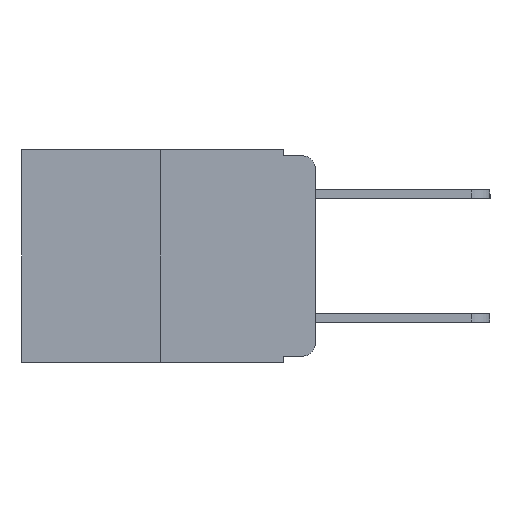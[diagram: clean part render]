
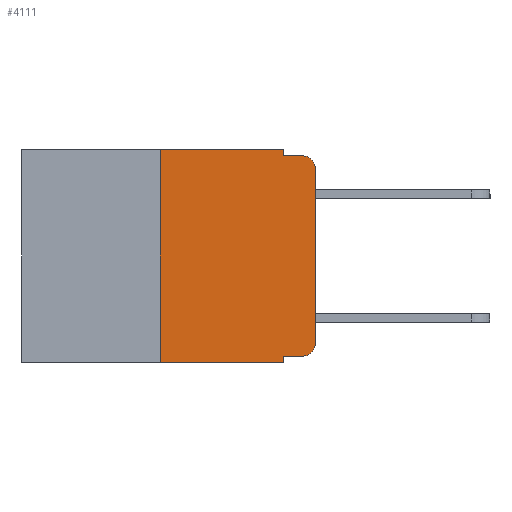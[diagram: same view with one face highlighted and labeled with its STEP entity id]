
A CAD part, left-side view. The second image highlights one B-rep face of the part: STEP entity #4111.
In plain terms, the highlighted planar face has unit normal (-1, 0, 0).
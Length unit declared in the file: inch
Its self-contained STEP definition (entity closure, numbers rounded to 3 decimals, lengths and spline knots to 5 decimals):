
#1461 = ORIENTED_EDGE ( 'NONE', *, *, #3324, .T. ) ;
#2060 = CARTESIAN_POINT ( 'NONE',  ( 0., 0.473, 0. ) ) ;
#2129 = VERTEX_POINT ( 'NONE', #2638 ) ;
#2429 = EDGE_CURVE ( 'NONE', #4318, #19544, #10494, .T. ) ;
#2447 = CARTESIAN_POINT ( 'NONE',  ( 0., 0.25, 0. ) ) ;
#2461 = ORIENTED_EDGE ( 'NONE', *, *, #3360, .F. ) ;
#2638 = CARTESIAN_POINT ( 'NONE',  ( 0., 0.02, -0.01 ) ) ;
#2941 = EDGE_CURVE ( 'NONE', #18041, #9579, #5008, .T. ) ;
#3286 = EDGE_CURVE ( 'NONE', #7197, #5409, #10718, .T. ) ;
#3324 = EDGE_CURVE ( 'NONE', #5409, #2129, #13878, .T. ) ;
#3356 = EDGE_CURVE ( 'NONE', #8829, #2129, #12909, .T. ) ;
#3360 = EDGE_CURVE ( 'NONE', #19544, #8829, #9157, .T. ) ;
#3364 = EDGE_CURVE ( 'NONE', #18041, #4318, #12422, .T. ) ;
#3393 = EDGE_CURVE ( 'NONE', #12695, #9579, #19845, .T. ) ;
#3397 = EDGE_CURVE ( 'NONE', #12695, #16929, #7543, .T. ) ;
#3403 = EDGE_CURVE ( 'NONE', #16929, #7197, #15535, .T. ) ;
#3817 = VECTOR ( 'NONE', #18798, 39.37008 ) ;
#4111 = ADVANCED_FACE ( 'NONE', ( #17070 ), #15646, .F. ) ;
#4318 = VERTEX_POINT ( 'NONE', #20542 ) ;
#4374 = EDGE_LOOP ( 'NONE', ( #9248, #1461, #4467, #2461, #11965, #5166, #5880, #7591, #19672, #5040 ) ) ;
#4393 = CARTESIAN_POINT ( 'NONE',  ( 0., 0.051, -0.01 ) ) ;
#4467 = ORIENTED_EDGE ( 'NONE', *, *, #3356, .F. ) ;
#4569 = CARTESIAN_POINT ( 'NONE',  ( 0., 0.051, 0. ) ) ;
#5008 = LINE ( 'NONE', #8054, #17343 ) ;
#5040 = ORIENTED_EDGE ( 'NONE', *, *, #3403, .T. ) ;
#5166 = ORIENTED_EDGE ( 'NONE', *, *, #3364, .F. ) ;
#5409 = VERTEX_POINT ( 'NONE', #11199 ) ;
#5774 = DIRECTION ( 'NONE',  ( 0., -1., 0. ) ) ;
#5880 = ORIENTED_EDGE ( 'NONE', *, *, #2941, .T. ) ;
#5908 = DIRECTION ( 'NONE',  ( 1., 0., 0. ) ) ;
#5954 = DIRECTION ( 'NONE',  ( 0., 0., 1. ) ) ;
#6114 = DIRECTION ( 'NONE',  ( -1., 0., 0. ) ) ;
#7197 = VERTEX_POINT ( 'NONE', #17632 ) ;
#7543 = LINE ( 'NONE', #8169, #19384 ) ;
#7591 = ORIENTED_EDGE ( 'NONE', *, *, #3393, .F. ) ;
#8025 = DIRECTION ( 'NONE',  ( 0., 0., 1. ) ) ;
#8054 = CARTESIAN_POINT ( 'NONE',  ( 0., 0.473, -0.343 ) ) ;
#8056 = VECTOR ( 'NONE', #8025, 39.37008 ) ;
#8169 = CARTESIAN_POINT ( 'NONE',  ( 0., 0.051, -0.333 ) ) ;
#8247 = DIRECTION ( 'NONE',  ( -1., 0., 0. ) ) ;
#8829 = VERTEX_POINT ( 'NONE', #20942 ) ;
#9157 = LINE ( 'NONE', #12878, #3817 ) ;
#9248 = ORIENTED_EDGE ( 'NONE', *, *, #3286, .T. ) ;
#9579 = VERTEX_POINT ( 'NONE', #18326 ) ;
#9850 = AXIS2_PLACEMENT_3D ( 'NONE', #17580, #8247, #19045 ) ;
#9942 = DIRECTION ( 'NONE',  ( 0., -1., 0. ) ) ;
#10494 = LINE ( 'NONE', #10959, #14647 ) ;
#10718 = LINE ( 'NONE', #15676, #18728 ) ;
#10959 = CARTESIAN_POINT ( 'NONE',  ( 0., 0.473, 0. ) ) ;
#11199 = CARTESIAN_POINT ( 'NONE',  ( 0., 0., -0.03 ) ) ;
#11469 = DIRECTION ( 'NONE',  ( 0., 0., -1. ) ) ;
#11965 = ORIENTED_EDGE ( 'NONE', *, *, #2429, .F. ) ;
#12422 = LINE ( 'NONE', #2447, #8056 ) ;
#12592 = CARTESIAN_POINT ( 'NONE',  ( 0., 0.051, 0. ) ) ;
#12695 = VERTEX_POINT ( 'NONE', #20252 ) ;
#12878 = CARTESIAN_POINT ( 'NONE',  ( 0., 0.051, 0. ) ) ;
#12884 = AXIS2_PLACEMENT_3D ( 'NONE', #2060, #5908, #17093 ) ;
#12909 = LINE ( 'NONE', #4393, #20702 ) ;
#13878 = CIRCLE ( 'NONE', #16419, 0.02 ) ;
#14647 = VECTOR ( 'NONE', #5774, 39.37008 ) ;
#15535 = CIRCLE ( 'NONE', #9850, 0.02 ) ;
#15646 = PLANE ( 'NONE',  #12884 ) ;
#15676 = CARTESIAN_POINT ( 'NONE',  ( 0., 0., 0. ) ) ;
#15806 = CARTESIAN_POINT ( 'NONE',  ( 0., 0.02, -0.03 ) ) ;
#15926 = DIRECTION ( 'NONE',  ( 0., -1., 0. ) ) ;
#15949 = DIRECTION ( 'NONE',  ( 0., -1., 0. ) ) ;
#15990 = VECTOR ( 'NONE', #11469, 39.37008 ) ;
#16102 = CARTESIAN_POINT ( 'NONE',  ( 0., 0.25, -0.343 ) ) ;
#16419 = AXIS2_PLACEMENT_3D ( 'NONE', #15806, #6114, #17256 ) ;
#16929 = VERTEX_POINT ( 'NONE', #18664 ) ;
#17070 = FACE_OUTER_BOUND ( 'NONE', #4374, .T. ) ;
#17093 = DIRECTION ( 'NONE',  ( 0., 0., -1. ) ) ;
#17256 = DIRECTION ( 'NONE',  ( 0., 0., -1. ) ) ;
#17343 = VECTOR ( 'NONE', #15949, 39.37008 ) ;
#17580 = CARTESIAN_POINT ( 'NONE',  ( 0., 0.02, -0.313 ) ) ;
#17632 = CARTESIAN_POINT ( 'NONE',  ( 0., 0., -0.313 ) ) ;
#18041 = VERTEX_POINT ( 'NONE', #16102 ) ;
#18326 = CARTESIAN_POINT ( 'NONE',  ( 0., 0.051, -0.343 ) ) ;
#18664 = CARTESIAN_POINT ( 'NONE',  ( 0., 0.02, -0.333 ) ) ;
#18728 = VECTOR ( 'NONE', #5954, 39.37008 ) ;
#18798 = DIRECTION ( 'NONE',  ( 0., 0., -1. ) ) ;
#19045 = DIRECTION ( 'NONE',  ( 0., 0., -1. ) ) ;
#19384 = VECTOR ( 'NONE', #9942, 39.37008 ) ;
#19544 = VERTEX_POINT ( 'NONE', #12592 ) ;
#19672 = ORIENTED_EDGE ( 'NONE', *, *, #3397, .T. ) ;
#19845 = LINE ( 'NONE', #4569, #15990 ) ;
#20252 = CARTESIAN_POINT ( 'NONE',  ( 0., 0.051, -0.333 ) ) ;
#20542 = CARTESIAN_POINT ( 'NONE',  ( 0., 0.25, 0. ) ) ;
#20702 = VECTOR ( 'NONE', #15926, 39.37008 ) ;
#20942 = CARTESIAN_POINT ( 'NONE',  ( 0., 0.051, -0.01 ) ) ;
